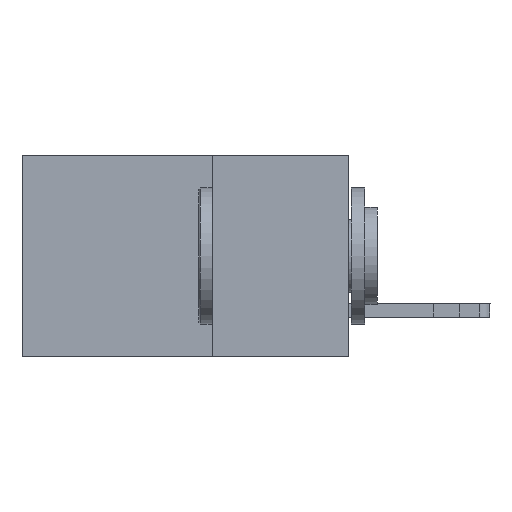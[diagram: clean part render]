
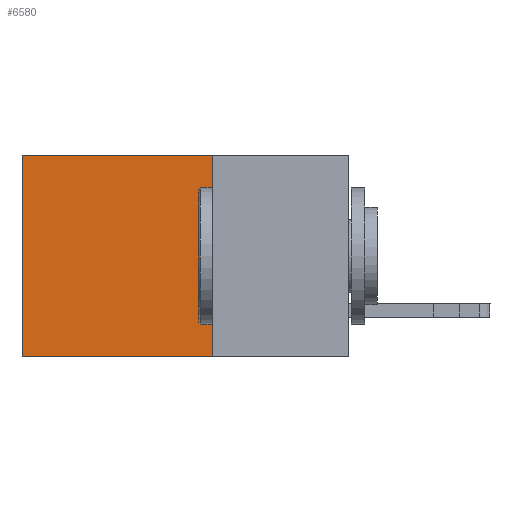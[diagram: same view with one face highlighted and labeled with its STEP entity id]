
A CAD part, left-side view. The second image highlights one B-rep face of the part: STEP entity #6580.
In plain terms, the highlighted planar face has unit normal (-1, 0, 0).
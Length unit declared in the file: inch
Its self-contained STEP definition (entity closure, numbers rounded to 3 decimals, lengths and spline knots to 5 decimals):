
#77 = VERTEX_POINT ( 'NONE', #4597 ) ;
#491 = LINE ( 'NONE', #9936, #10722 ) ;
#661 = EDGE_CURVE ( 'NONE', #3639, #6203, #12663, .T. ) ;
#1155 = CARTESIAN_POINT ( 'NONE',  ( 0.2615, 0.25, -0.37 ) ) ;
#1327 = ORIENTED_EDGE ( 'NONE', *, *, #7877, .T. ) ;
#1426 = DIRECTION ( 'NONE',  ( 0., 0., -1. ) ) ;
#1469 = EDGE_CURVE ( 'NONE', #11610, #6203, #4106, .T. ) ;
#2090 = LINE ( 'NONE', #11263, #10020 ) ;
#2851 = DIRECTION ( 'NONE',  ( 1., 0., 0. ) ) ;
#3639 = VERTEX_POINT ( 'NONE', #4796 ) ;
#3791 = VECTOR ( 'NONE', #11985, 39.37008 ) ;
#3951 = ORIENTED_EDGE ( 'NONE', *, *, #1469, .T. ) ;
#4106 = LINE ( 'NONE', #4201, #3791 ) ;
#4201 = CARTESIAN_POINT ( 'NONE',  ( 0.2615, 0.6, -0.37 ) ) ;
#4597 = CARTESIAN_POINT ( 'NONE',  ( 0.2615, 0.25, 0. ) ) ;
#4796 = CARTESIAN_POINT ( 'NONE',  ( 0.2615, 0.25, -0.37 ) ) ;
#4813 = PLANE ( 'NONE',  #8158 ) ;
#5091 = EDGE_LOOP ( 'NONE', ( #3951, #9846, #7849, #1327 ) ) ;
#6203 = VERTEX_POINT ( 'NONE', #9268 ) ;
#6580 = ADVANCED_FACE ( 'NONE', ( #9852 ), #4813, .F. ) ;
#7849 = ORIENTED_EDGE ( 'NONE', *, *, #12775, .F. ) ;
#7877 = EDGE_CURVE ( 'NONE', #77, #11610, #491, .T. ) ;
#8158 = AXIS2_PLACEMENT_3D ( 'NONE', #8846, #2851, #9808 ) ;
#8846 = CARTESIAN_POINT ( 'NONE',  ( 0.2615, 0.25, -0.37 ) ) ;
#9268 = CARTESIAN_POINT ( 'NONE',  ( 0.2615, 0.6, -0.37 ) ) ;
#9808 = DIRECTION ( 'NONE',  ( 0., 0., -1. ) ) ;
#9846 = ORIENTED_EDGE ( 'NONE', *, *, #661, .F. ) ;
#9852 = FACE_OUTER_BOUND ( 'NONE', #5091, .T. ) ;
#9936 = CARTESIAN_POINT ( 'NONE',  ( 0.2615, 0.25, 0. ) ) ;
#10020 = VECTOR ( 'NONE', #1426, 39.37008 ) ;
#10135 = VECTOR ( 'NONE', #11583, 39.37008 ) ;
#10531 = CARTESIAN_POINT ( 'NONE',  ( 0.2615, 0.6, 0. ) ) ;
#10722 = VECTOR ( 'NONE', #10901, 39.37008 ) ;
#10901 = DIRECTION ( 'NONE',  ( 0., 1., 0. ) ) ;
#11263 = CARTESIAN_POINT ( 'NONE',  ( 0.2615, 0.25, -0.37 ) ) ;
#11583 = DIRECTION ( 'NONE',  ( 0., 1., 0. ) ) ;
#11610 = VERTEX_POINT ( 'NONE', #10531 ) ;
#11985 = DIRECTION ( 'NONE',  ( 0., 0., -1. ) ) ;
#12663 = LINE ( 'NONE', #1155, #10135 ) ;
#12775 = EDGE_CURVE ( 'NONE', #77, #3639, #2090, .T. ) ;
